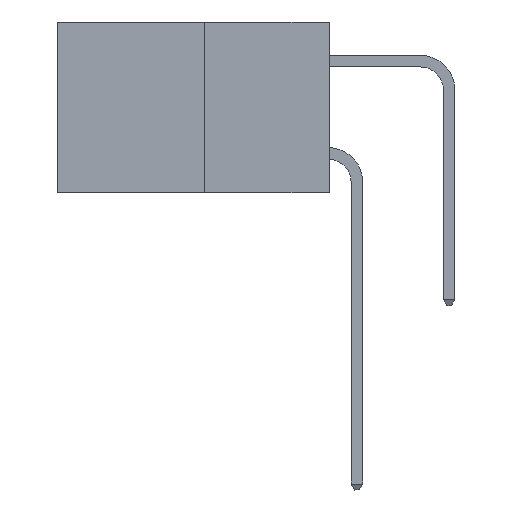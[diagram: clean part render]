
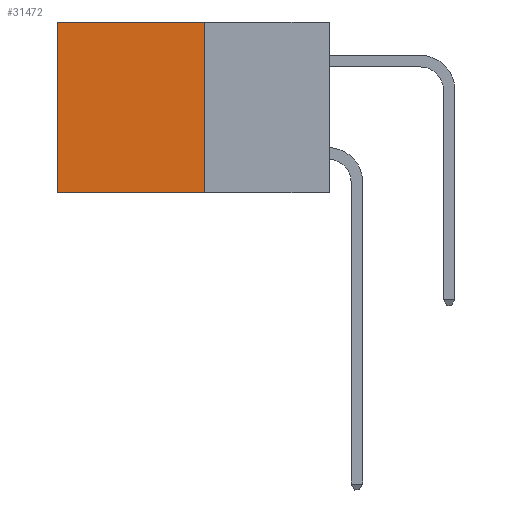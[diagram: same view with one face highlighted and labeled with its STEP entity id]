
A CAD part, left-side view. The second image highlights one B-rep face of the part: STEP entity #31472.
In plain terms, the highlighted planar face has unit normal (-1, 0, 0).
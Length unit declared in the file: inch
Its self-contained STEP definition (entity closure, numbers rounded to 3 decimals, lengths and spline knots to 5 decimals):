
#2802 = VECTOR ( 'NONE', #25113, 39.37008 ) ;
#3168 = DIRECTION ( 'NONE',  ( 0., 1., 0. ) ) ;
#3849 = PLANE ( 'NONE',  #8771 ) ;
#6435 = VERTEX_POINT ( 'NONE', #18094 ) ;
#8771 = AXIS2_PLACEMENT_3D ( 'NONE', #9152, #33452, #9263 ) ;
#9152 = CARTESIAN_POINT ( 'NONE',  ( 0.277, 0.27, -0.37 ) ) ;
#9263 = DIRECTION ( 'NONE',  ( 0., 0., -1. ) ) ;
#9489 = EDGE_LOOP ( 'NONE', ( #17885, #26323, #11106, #20276 ) ) ;
#9937 = FACE_OUTER_BOUND ( 'NONE', #9489, .T. ) ;
#10836 = DIRECTION ( 'NONE',  ( 0., 0., -1. ) ) ;
#10858 = VECTOR ( 'NONE', #25002, 39.37008 ) ;
#11106 = ORIENTED_EDGE ( 'NONE', *, *, #18379, .F. ) ;
#11414 = LINE ( 'NONE', #18977, #32191 ) ;
#11680 = LINE ( 'NONE', #24875, #10858 ) ;
#13065 = CARTESIAN_POINT ( 'NONE',  ( 0.277, 0.27, 0. ) ) ;
#13440 = CARTESIAN_POINT ( 'NONE',  ( 0.277, 0.59, -0.37 ) ) ;
#13911 = CARTESIAN_POINT ( 'NONE',  ( 0.277, 0.27, 0. ) ) ;
#16080 = VERTEX_POINT ( 'NONE', #13440 ) ;
#16484 = VERTEX_POINT ( 'NONE', #33828 ) ;
#17885 = ORIENTED_EDGE ( 'NONE', *, *, #22917, .T. ) ;
#18094 = CARTESIAN_POINT ( 'NONE',  ( 0.277, 0.27, -0.37 ) ) ;
#18334 = EDGE_CURVE ( 'NONE', #32849, #16484, #26265, .T. ) ;
#18337 = EDGE_CURVE ( 'NONE', #6435, #16080, #11680, .T. ) ;
#18379 = EDGE_CURVE ( 'NONE', #32849, #6435, #32442, .T. ) ;
#18977 = CARTESIAN_POINT ( 'NONE',  ( 0.277, 0.59, -0.37 ) ) ;
#20276 = ORIENTED_EDGE ( 'NONE', *, *, #18334, .T. ) ;
#22917 = EDGE_CURVE ( 'NONE', #16484, #16080, #11414, .T. ) ;
#24875 = CARTESIAN_POINT ( 'NONE',  ( 0.277, 0.27, -0.37 ) ) ;
#25002 = DIRECTION ( 'NONE',  ( 0., 1., 0. ) ) ;
#25113 = DIRECTION ( 'NONE',  ( 0., 0., -1. ) ) ;
#25416 = VECTOR ( 'NONE', #3168, 39.37008 ) ;
#26265 = LINE ( 'NONE', #13911, #25416 ) ;
#26323 = ORIENTED_EDGE ( 'NONE', *, *, #18337, .F. ) ;
#31472 = ADVANCED_FACE ( 'NONE', ( #9937 ), #3849, .F. ) ;
#32191 = VECTOR ( 'NONE', #10836, 39.37008 ) ;
#32442 = LINE ( 'NONE', #32933, #2802 ) ;
#32849 = VERTEX_POINT ( 'NONE', #13065 ) ;
#32933 = CARTESIAN_POINT ( 'NONE',  ( 0.277, 0.27, -0.37 ) ) ;
#33452 = DIRECTION ( 'NONE',  ( 1., 0., 0. ) ) ;
#33828 = CARTESIAN_POINT ( 'NONE',  ( 0.277, 0.59, 0. ) ) ;
